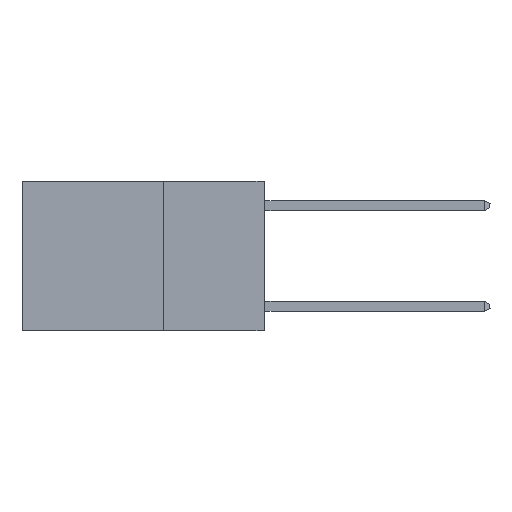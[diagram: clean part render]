
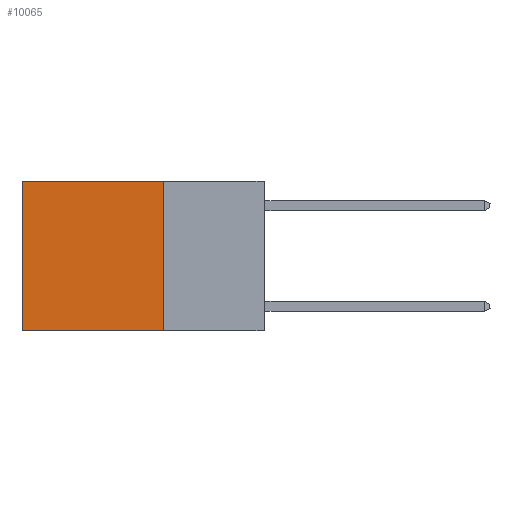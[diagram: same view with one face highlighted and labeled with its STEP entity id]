
A CAD part, left-side view. The second image highlights one B-rep face of the part: STEP entity #10065.
In plain terms, the highlighted planar face has unit normal (-1, 0, 0).
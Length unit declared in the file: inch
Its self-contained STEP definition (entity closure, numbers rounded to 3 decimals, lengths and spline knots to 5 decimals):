
#399 = EDGE_CURVE ( 'NONE', #10595, #9286, #5263, .T. ) ;
#618 = DIRECTION ( 'NONE',  ( 0., 1., 0. ) ) ;
#663 = VECTOR ( 'NONE', #9943, 39.37008 ) ;
#1028 = CARTESIAN_POINT ( 'NONE',  ( 0.2625, 0.25, -0.37 ) ) ;
#1147 = ORIENTED_EDGE ( 'NONE', *, *, #8154, .T. ) ;
#1485 = LINE ( 'NONE', #4837, #7797 ) ;
#1567 = PLANE ( 'NONE',  #9415 ) ;
#1954 = CARTESIAN_POINT ( 'NONE',  ( 0.2625, 0.25, 0. ) ) ;
#2184 = CARTESIAN_POINT ( 'NONE',  ( 0.2625, 0.25, 0. ) ) ;
#2968 = VERTEX_POINT ( 'NONE', #1954 ) ;
#3159 = ORIENTED_EDGE ( 'NONE', *, *, #399, .F. ) ;
#3207 = DIRECTION ( 'NONE',  ( 0., 0., -1. ) ) ;
#4402 = CARTESIAN_POINT ( 'NONE',  ( 0.2625, 0.6, 0. ) ) ;
#4759 = EDGE_CURVE ( 'NONE', #2968, #10595, #1485, .T. ) ;
#4837 = CARTESIAN_POINT ( 'NONE',  ( 0.2625, 0.25, 0. ) ) ;
#5071 = CARTESIAN_POINT ( 'NONE',  ( 0.2625, 0.6, 0. ) ) ;
#5263 = LINE ( 'NONE', #5372, #6671 ) ;
#5372 = CARTESIAN_POINT ( 'NONE',  ( 0.2625, 0.25, -0.37 ) ) ;
#5729 = ORIENTED_EDGE ( 'NONE', *, *, #4759, .F. ) ;
#6176 = EDGE_LOOP ( 'NONE', ( #6226, #3159, #5729, #1147 ) ) ;
#6226 = ORIENTED_EDGE ( 'NONE', *, *, #8816, .T. ) ;
#6410 = DIRECTION ( 'NONE',  ( 0., 0., -1. ) ) ;
#6541 = FACE_OUTER_BOUND ( 'NONE', #6176, .T. ) ;
#6671 = VECTOR ( 'NONE', #8712, 39.37008 ) ;
#7797 = VECTOR ( 'NONE', #6410, 39.37008 ) ;
#8093 = LINE ( 'NONE', #2184, #8360 ) ;
#8154 = EDGE_CURVE ( 'NONE', #2968, #8530, #8093, .T. ) ;
#8286 = LINE ( 'NONE', #5071, #663 ) ;
#8360 = VECTOR ( 'NONE', #618, 39.37008 ) ;
#8530 = VERTEX_POINT ( 'NONE', #4402 ) ;
#8712 = DIRECTION ( 'NONE',  ( 0., 1., 0. ) ) ;
#8816 = EDGE_CURVE ( 'NONE', #8530, #9286, #8286, .T. ) ;
#9065 = DIRECTION ( 'NONE',  ( 1., 0., 0. ) ) ;
#9089 = CARTESIAN_POINT ( 'NONE',  ( 0.2625, 0.6, -0.37 ) ) ;
#9286 = VERTEX_POINT ( 'NONE', #9089 ) ;
#9415 = AXIS2_PLACEMENT_3D ( 'NONE', #10109, #9065, #3207 ) ;
#9943 = DIRECTION ( 'NONE',  ( 0., 0., -1. ) ) ;
#10065 = ADVANCED_FACE ( 'NONE', ( #6541 ), #1567, .F. ) ;
#10109 = CARTESIAN_POINT ( 'NONE',  ( 0.2625, 0.25, 0. ) ) ;
#10595 = VERTEX_POINT ( 'NONE', #1028 ) ;
